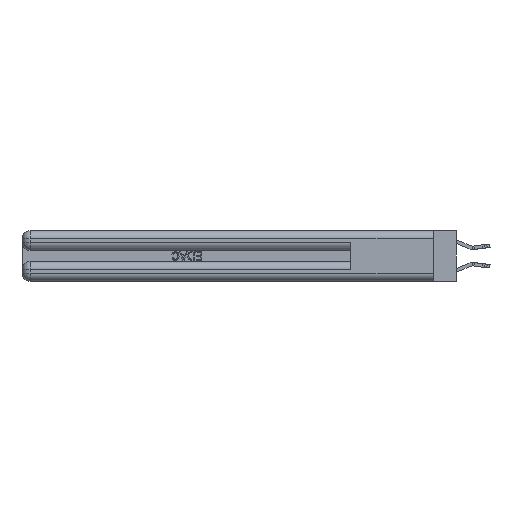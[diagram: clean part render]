
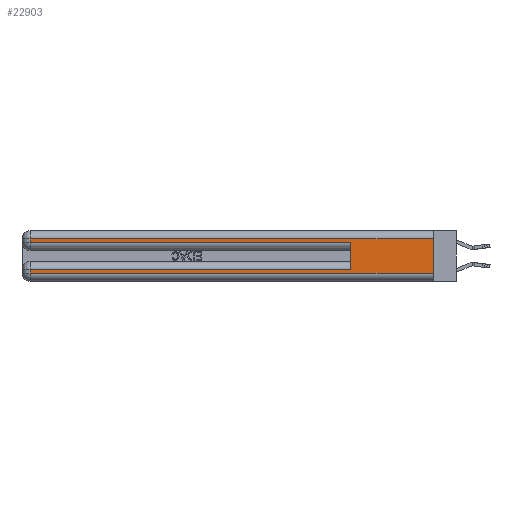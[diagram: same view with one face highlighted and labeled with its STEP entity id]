
A CAD part, left-side view. The second image highlights one B-rep face of the part: STEP entity #22903.
In plain terms, the highlighted planar face has unit normal (-1, 0, 0).
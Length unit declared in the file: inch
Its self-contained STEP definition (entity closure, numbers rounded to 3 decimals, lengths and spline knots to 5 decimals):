
#498 = CARTESIAN_POINT ( 'NONE',  ( 0., 2.94, 0.085 ) ) ;
#1402 = CARTESIAN_POINT ( 'NONE',  ( 0., 0., 0.37 ) ) ;
#1772 = LINE ( 'NONE', #17573, #5014 ) ;
#1792 = ORIENTED_EDGE ( 'NONE', *, *, #12988, .F. ) ;
#2147 = DIRECTION ( 'NONE',  ( 0., 0., 1. ) ) ;
#2825 = AXIS2_PLACEMENT_3D ( 'NONE', #1402, #33895, #9579 ) ;
#3914 = VERTEX_POINT ( 'NONE', #498 ) ;
#3954 = CARTESIAN_POINT ( 'NONE',  ( 0., 2.94, 0.06 ) ) ;
#5014 = VECTOR ( 'NONE', #12584, 39.37008 ) ;
#5079 = EDGE_CURVE ( 'NONE', #3914, #24147, #12370, .T. ) ;
#5581 = DIRECTION ( 'NONE',  ( 0., -1., 0. ) ) ;
#6239 = DIRECTION ( 'NONE',  ( 0., 0., -1. ) ) ;
#6980 = EDGE_LOOP ( 'NONE', ( #1792, #10678, #20124, #32312, #12461, #7545, #25610, #13230 ) ) ;
#7545 = ORIENTED_EDGE ( 'NONE', *, *, #29245, .T. ) ;
#8216 = DIRECTION ( 'NONE',  ( 0., 1., 0. ) ) ;
#8233 = LINE ( 'NONE', #19067, #11089 ) ;
#8387 = LINE ( 'NONE', #32554, #9569 ) ;
#8496 = VERTEX_POINT ( 'NONE', #28476 ) ;
#9220 = CARTESIAN_POINT ( 'NONE',  ( 0., 0.6, 0.085 ) ) ;
#9543 = CARTESIAN_POINT ( 'NONE',  ( 0., 2.94, 0.37 ) ) ;
#9569 = VECTOR ( 'NONE', #8216, 39.37008 ) ;
#9579 = DIRECTION ( 'NONE',  ( 0., 0., -1. ) ) ;
#9690 = EDGE_CURVE ( 'NONE', #14769, #11371, #28135, .T. ) ;
#10355 = VECTOR ( 'NONE', #6239, 39.37008 ) ;
#10678 = ORIENTED_EDGE ( 'NONE', *, *, #9690, .T. ) ;
#10702 = CARTESIAN_POINT ( 'NONE',  ( 0., 0., 0.31 ) ) ;
#10795 = VECTOR ( 'NONE', #17535, 39.37008 ) ;
#11089 = VECTOR ( 'NONE', #5581, 39.37008 ) ;
#11371 = VERTEX_POINT ( 'NONE', #23305 ) ;
#11478 = CARTESIAN_POINT ( 'NONE',  ( 0., 0.6, 0.145 ) ) ;
#11531 = VECTOR ( 'NONE', #2147, 39.37008 ) ;
#11554 = CARTESIAN_POINT ( 'NONE',  ( 0., 0., 0.37 ) ) ;
#12076 = LINE ( 'NONE', #11554, #10355 ) ;
#12130 = CARTESIAN_POINT ( 'NONE',  ( 0., 2.94, 0.285 ) ) ;
#12370 = LINE ( 'NONE', #9543, #10795 ) ;
#12461 = ORIENTED_EDGE ( 'NONE', *, *, #13739, .F. ) ;
#12584 = DIRECTION ( 'NONE',  ( 0., -1., 0. ) ) ;
#12988 = EDGE_CURVE ( 'NONE', #14769, #31296, #12076, .T. ) ;
#13063 = LINE ( 'NONE', #24251, #19929 ) ;
#13230 = ORIENTED_EDGE ( 'NONE', *, *, #18458, .T. ) ;
#13739 = EDGE_CURVE ( 'NONE', #21525, #8496, #15090, .T. ) ;
#14769 = VERTEX_POINT ( 'NONE', #10702 ) ;
#15090 = LINE ( 'NONE', #11478, #11531 ) ;
#16251 = DIRECTION ( 'NONE',  ( 0., 0., -1. ) ) ;
#16759 = CARTESIAN_POINT ( 'NONE',  ( 0., 0., 0.06 ) ) ;
#17486 = DIRECTION ( 'NONE',  ( 0., 1., 0. ) ) ;
#17535 = DIRECTION ( 'NONE',  ( 0., 0., -1. ) ) ;
#17573 = CARTESIAN_POINT ( 'NONE',  ( 0., 0., 0.285 ) ) ;
#18458 = EDGE_CURVE ( 'NONE', #24147, #31296, #8233, .T. ) ;
#19067 = CARTESIAN_POINT ( 'NONE',  ( 0., 0., 0.06 ) ) ;
#19929 = VECTOR ( 'NONE', #16251, 39.37008 ) ;
#20124 = ORIENTED_EDGE ( 'NONE', *, *, #32455, .T. ) ;
#20223 = PLANE ( 'NONE',  #2825 ) ;
#21525 = VERTEX_POINT ( 'NONE', #9220 ) ;
#22903 = ADVANCED_FACE ( 'NONE', ( #25725 ), #20223, .F. ) ;
#23305 = CARTESIAN_POINT ( 'NONE',  ( 0., 2.94, 0.31 ) ) ;
#23744 = VECTOR ( 'NONE', #17486, 39.37008 ) ;
#24147 = VERTEX_POINT ( 'NONE', #3954 ) ;
#24251 = CARTESIAN_POINT ( 'NONE',  ( 0., 2.94, 0.37 ) ) ;
#25472 = CARTESIAN_POINT ( 'NONE',  ( 0., 0., 0.31 ) ) ;
#25610 = ORIENTED_EDGE ( 'NONE', *, *, #5079, .T. ) ;
#25725 = FACE_OUTER_BOUND ( 'NONE', #6980, .T. ) ;
#26544 = VERTEX_POINT ( 'NONE', #12130 ) ;
#28135 = LINE ( 'NONE', #25472, #23744 ) ;
#28476 = CARTESIAN_POINT ( 'NONE',  ( 0., 0.6, 0.285 ) ) ;
#28604 = EDGE_CURVE ( 'NONE', #26544, #8496, #1772, .T. ) ;
#29245 = EDGE_CURVE ( 'NONE', #21525, #3914, #8387, .T. ) ;
#31296 = VERTEX_POINT ( 'NONE', #16759 ) ;
#32312 = ORIENTED_EDGE ( 'NONE', *, *, #28604, .T. ) ;
#32455 = EDGE_CURVE ( 'NONE', #11371, #26544, #13063, .T. ) ;
#32554 = CARTESIAN_POINT ( 'NONE',  ( 0., 0., 0.085 ) ) ;
#33895 = DIRECTION ( 'NONE',  ( 1., 0., 0. ) ) ;
